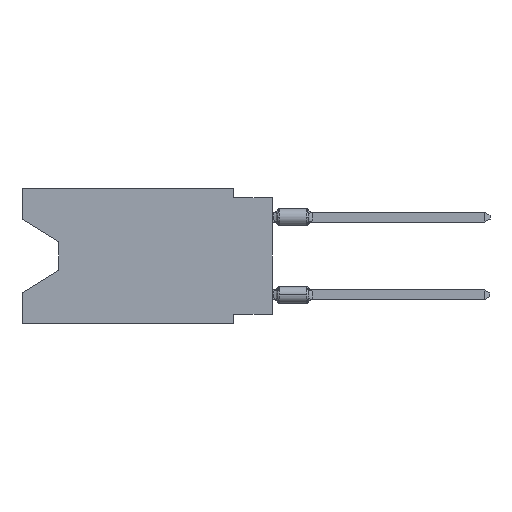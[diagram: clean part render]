
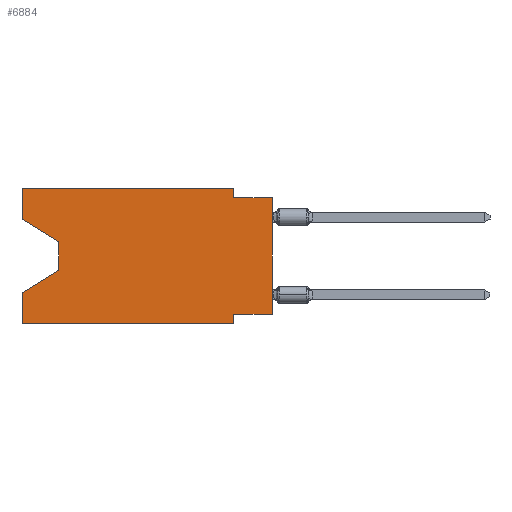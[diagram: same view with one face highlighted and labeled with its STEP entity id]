
A CAD part, left-side view. The second image highlights one B-rep face of the part: STEP entity #6884.
In plain terms, the highlighted planar face has unit normal (-1, 0, 0).
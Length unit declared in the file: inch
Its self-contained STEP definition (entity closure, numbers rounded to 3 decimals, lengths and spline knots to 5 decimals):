
#432 = EDGE_CURVE ( 'NONE', #6979, #36840, #31461, .T. ) ;
#477 = VERTEX_POINT ( 'NONE', #11176 ) ;
#880 = EDGE_CURVE ( 'NONE', #15112, #36840, #25422, .T. ) ;
#1024 = CARTESIAN_POINT ( 'NONE',  ( 0., 0.1, 0. ) ) ;
#2238 = VECTOR ( 'NONE', #18198, 39.37008 ) ;
#3405 = CARTESIAN_POINT ( 'NONE',  ( 0., 0.55, -0.212 ) ) ;
#3641 = CARTESIAN_POINT ( 'NONE',  ( 0., 0.645, 0. ) ) ;
#4843 = ORIENTED_EDGE ( 'NONE', *, *, #432, .T. ) ;
#5501 = CARTESIAN_POINT ( 'NONE',  ( 0., 0., 0. ) ) ;
#5940 = LINE ( 'NONE', #31522, #37141 ) ;
#6112 = DIRECTION ( 'NONE',  ( 1., 0., 0. ) ) ;
#6473 = VERTEX_POINT ( 'NONE', #21953 ) ;
#6487 = DIRECTION ( 'NONE',  ( 0., 0., -1. ) ) ;
#6618 = CARTESIAN_POINT ( 'NONE',  ( 0., 0.645, -0.26975 ) ) ;
#6730 = VECTOR ( 'NONE', #24708, 39.37008 ) ;
#6884 = ADVANCED_FACE ( 'NONE', ( #24951 ), #31702, .F. ) ;
#6979 = VERTEX_POINT ( 'NONE', #19593 ) ;
#7350 = CARTESIAN_POINT ( 'NONE',  ( 0., 0.645, -0.08025 ) ) ;
#7395 = VECTOR ( 'NONE', #26742, 39.37008 ) ;
#7423 = EDGE_CURVE ( 'NONE', #29829, #6473, #27334, .T. ) ;
#10442 = CARTESIAN_POINT ( 'NONE',  ( 0., 0.1, -0.325 ) ) ;
#11042 = ORIENTED_EDGE ( 'NONE', *, *, #7423, .F. ) ;
#11176 = CARTESIAN_POINT ( 'NONE',  ( 0., 0., -0.325 ) ) ;
#11460 = LINE ( 'NONE', #5501, #2238 ) ;
#11501 = EDGE_CURVE ( 'NONE', #477, #34255, #31438, .T. ) ;
#11510 = CARTESIAN_POINT ( 'NONE',  ( 0., 0.645, 0. ) ) ;
#11570 = LINE ( 'NONE', #17340, #35277 ) ;
#11691 = DIRECTION ( 'NONE',  ( 0., -1., 0. ) ) ;
#11725 = LINE ( 'NONE', #15586, #26700 ) ;
#12523 = CARTESIAN_POINT ( 'NONE',  ( 0., 0.1, -0.025 ) ) ;
#13240 = ORIENTED_EDGE ( 'NONE', *, *, #32068, .T. ) ;
#13791 = VERTEX_POINT ( 'NONE', #1024 ) ;
#15112 = VERTEX_POINT ( 'NONE', #20710 ) ;
#15586 = CARTESIAN_POINT ( 'NONE',  ( 0., 0.55, -0.138 ) ) ;
#16129 = DIRECTION ( 'NONE',  ( 0., 0., -1. ) ) ;
#16433 = VECTOR ( 'NONE', #22370, 39.37008 ) ;
#16517 = DIRECTION ( 'NONE',  ( 0., 0.855, -0.519 ) ) ;
#16646 = EDGE_CURVE ( 'NONE', #34697, #39651, #38278, .T. ) ;
#16881 = ORIENTED_EDGE ( 'NONE', *, *, #16646, .T. ) ;
#17340 = CARTESIAN_POINT ( 'NONE',  ( 0., 0.645, -0.35 ) ) ;
#18053 = EDGE_CURVE ( 'NONE', #34697, #35970, #5940, .T. ) ;
#18198 = DIRECTION ( 'NONE',  ( 0., 0., 1. ) ) ;
#18477 = EDGE_CURVE ( 'NONE', #34255, #22494, #28193, .T. ) ;
#19203 = EDGE_CURVE ( 'NONE', #35970, #13791, #26537, .T. ) ;
#19348 = DIRECTION ( 'NONE',  ( 0., 0., -1. ) ) ;
#19593 = CARTESIAN_POINT ( 'NONE',  ( 0., 0.55, -0.212 ) ) ;
#20121 = EDGE_CURVE ( 'NONE', #13791, #29829, #20177, .T. ) ;
#20177 = LINE ( 'NONE', #35755, #29980 ) ;
#20609 = CARTESIAN_POINT ( 'NONE',  ( 0., 0., -0.025 ) ) ;
#20672 = ORIENTED_EDGE ( 'NONE', *, *, #18053, .F. ) ;
#20710 = CARTESIAN_POINT ( 'NONE',  ( 0., 0.645, -0.35 ) ) ;
#21646 = CARTESIAN_POINT ( 'NONE',  ( 0., 0., -0.325 ) ) ;
#21953 = CARTESIAN_POINT ( 'NONE',  ( 0., 0., -0.025 ) ) ;
#22099 = ORIENTED_EDGE ( 'NONE', *, *, #33537, .T. ) ;
#22370 = DIRECTION ( 'NONE',  ( 0., 0., 1. ) ) ;
#22494 = VERTEX_POINT ( 'NONE', #24310 ) ;
#23011 = VECTOR ( 'NONE', #28850, 39.37008 ) ;
#24230 = DIRECTION ( 'NONE',  ( 0., 0., -1. ) ) ;
#24310 = CARTESIAN_POINT ( 'NONE',  ( 0., 0.1, -0.35 ) ) ;
#24343 = CARTESIAN_POINT ( 'NONE',  ( 0., 0.1, -0.35 ) ) ;
#24708 = DIRECTION ( 'NONE',  ( 0., 1., 0. ) ) ;
#24951 = FACE_OUTER_BOUND ( 'NONE', #33914, .T. ) ;
#24990 = DIRECTION ( 'NONE',  ( 0., 0., 1. ) ) ;
#25028 = AXIS2_PLACEMENT_3D ( 'NONE', #3641, #6112, #16129 ) ;
#25422 = LINE ( 'NONE', #37905, #16433 ) ;
#26537 = LINE ( 'NONE', #11510, #38371 ) ;
#26700 = VECTOR ( 'NONE', #24230, 39.37008 ) ;
#26742 = DIRECTION ( 'NONE',  ( 0., -1., 0. ) ) ;
#26949 = DIRECTION ( 'NONE',  ( 0., -1., 0. ) ) ;
#27334 = LINE ( 'NONE', #20609, #7395 ) ;
#27348 = VECTOR ( 'NONE', #6487, 39.37008 ) ;
#28193 = LINE ( 'NONE', #24343, #27348 ) ;
#28850 = DIRECTION ( 'NONE',  ( 0., -0.855, -0.519 ) ) ;
#29829 = VERTEX_POINT ( 'NONE', #12523 ) ;
#29980 = VECTOR ( 'NONE', #19348, 39.37008 ) ;
#30648 = EDGE_CURVE ( 'NONE', #477, #6473, #11460, .T. ) ;
#30679 = ORIENTED_EDGE ( 'NONE', *, *, #11501, .F. ) ;
#31038 = ORIENTED_EDGE ( 'NONE', *, *, #880, .F. ) ;
#31438 = LINE ( 'NONE', #21646, #6730 ) ;
#31461 = LINE ( 'NONE', #3405, #38762 ) ;
#31522 = CARTESIAN_POINT ( 'NONE',  ( 0., 0.645, 0. ) ) ;
#31702 = PLANE ( 'NONE',  #25028 ) ;
#31874 = ORIENTED_EDGE ( 'NONE', *, *, #18477, .F. ) ;
#32068 = EDGE_CURVE ( 'NONE', #39651, #6979, #11725, .T. ) ;
#33537 = EDGE_CURVE ( 'NONE', #15112, #22494, #11570, .T. ) ;
#33914 = EDGE_LOOP ( 'NONE', ( #16881, #13240, #4843, #31038, #22099, #31874, #30679, #35319, #11042, #39896, #35701, #20672 ) ) ;
#34255 = VERTEX_POINT ( 'NONE', #10442 ) ;
#34630 = CARTESIAN_POINT ( 'NONE',  ( 0., 0.645, 0. ) ) ;
#34697 = VERTEX_POINT ( 'NONE', #35612 ) ;
#35277 = VECTOR ( 'NONE', #26949, 39.37008 ) ;
#35319 = ORIENTED_EDGE ( 'NONE', *, *, #30648, .T. ) ;
#35612 = CARTESIAN_POINT ( 'NONE',  ( 0., 0.645, -0.08025 ) ) ;
#35701 = ORIENTED_EDGE ( 'NONE', *, *, #19203, .F. ) ;
#35755 = CARTESIAN_POINT ( 'NONE',  ( 0., 0.1, 0. ) ) ;
#35970 = VERTEX_POINT ( 'NONE', #34630 ) ;
#36840 = VERTEX_POINT ( 'NONE', #6618 ) ;
#37141 = VECTOR ( 'NONE', #24990, 39.37008 ) ;
#37336 = CARTESIAN_POINT ( 'NONE',  ( 0., 0.55, -0.138 ) ) ;
#37905 = CARTESIAN_POINT ( 'NONE',  ( 0., 0.645, 0. ) ) ;
#38278 = LINE ( 'NONE', #7350, #23011 ) ;
#38371 = VECTOR ( 'NONE', #11691, 39.37008 ) ;
#38762 = VECTOR ( 'NONE', #16517, 39.37008 ) ;
#39651 = VERTEX_POINT ( 'NONE', #37336 ) ;
#39896 = ORIENTED_EDGE ( 'NONE', *, *, #20121, .F. ) ;
